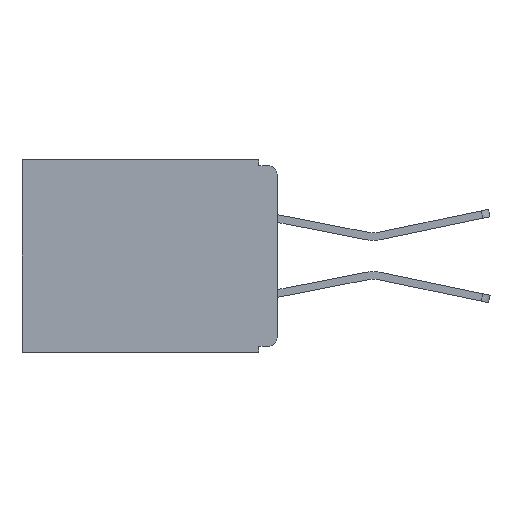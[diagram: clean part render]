
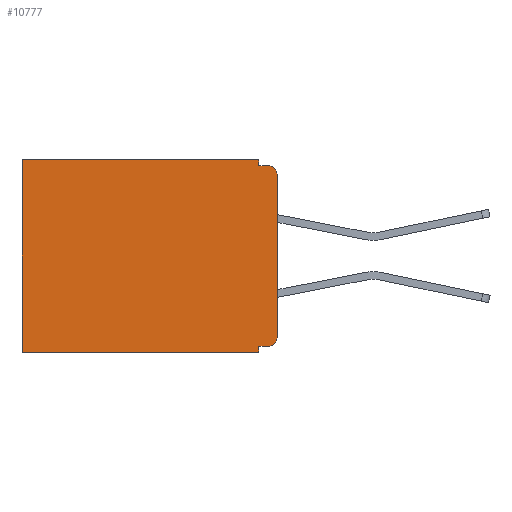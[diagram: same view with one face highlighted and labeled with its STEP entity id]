
A CAD part, left-side view. The second image highlights one B-rep face of the part: STEP entity #10777.
In plain terms, the highlighted planar face has unit normal (-1, 0, 0).
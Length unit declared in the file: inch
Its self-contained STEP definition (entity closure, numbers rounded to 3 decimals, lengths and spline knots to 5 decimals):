
#31 = CARTESIAN_POINT ( 'NONE',  ( 0.3, 0.015, -0.32 ) ) ;
#32 = EDGE_CURVE ( 'NONE', #7214, #6674, #7063, .T. ) ;
#183 = EDGE_CURVE ( 'NONE', #6575, #789, #5731, .T. ) ;
#282 = EDGE_CURVE ( 'NONE', #1045, #8537, #10183, .T. ) ;
#474 = DIRECTION ( 'NONE',  ( 0., 0., -1. ) ) ;
#475 = ORIENTED_EDGE ( 'NONE', *, *, #32, .T. ) ;
#490 = VECTOR ( 'NONE', #5329, 39.37008 ) ;
#765 = LINE ( 'NONE', #10491, #2820 ) ;
#789 = VERTEX_POINT ( 'NONE', #7204 ) ;
#797 = CARTESIAN_POINT ( 'NONE',  ( 0.3, 0., -0.33 ) ) ;
#808 = CARTESIAN_POINT ( 'NONE',  ( 0.3, 0., -0.025 ) ) ;
#1029 = FACE_OUTER_BOUND ( 'NONE', #3842, .T. ) ;
#1045 = VERTEX_POINT ( 'NONE', #3556 ) ;
#1159 = EDGE_CURVE ( 'NONE', #8537, #3041, #9257, .T. ) ;
#1324 = VECTOR ( 'NONE', #3701, 39.37008 ) ;
#1731 = EDGE_CURVE ( 'NONE', #2744, #3041, #5409, .T. ) ;
#2053 = EDGE_CURVE ( 'NONE', #1045, #8242, #10256, .T. ) ;
#2115 = EDGE_CURVE ( 'NONE', #4484, #2744, #765, .T. ) ;
#2306 = ORIENTED_EDGE ( 'NONE', *, *, #183, .T. ) ;
#2744 = VERTEX_POINT ( 'NONE', #6835 ) ;
#2820 = VECTOR ( 'NONE', #8658, 39.37008 ) ;
#3041 = VERTEX_POINT ( 'NONE', #7373 ) ;
#3066 = LINE ( 'NONE', #4452, #490 ) ;
#3301 = ORIENTED_EDGE ( 'NONE', *, *, #1731, .F. ) ;
#3378 = DIRECTION ( 'NONE',  ( 0., 1., 0. ) ) ;
#3556 = CARTESIAN_POINT ( 'NONE',  ( 0.3, 0.031, 0. ) ) ;
#3606 = ORIENTED_EDGE ( 'NONE', *, *, #2053, .F. ) ;
#3701 = DIRECTION ( 'NONE',  ( 0., 0., -1. ) ) ;
#3842 = EDGE_LOOP ( 'NONE', ( #9832, #475, #7612, #3606, #7212, #6824, #3301, #7018, #8519, #2306 ) ) ;
#3924 = PLANE ( 'NONE',  #8973 ) ;
#4018 = LINE ( 'NONE', #4693, #6080 ) ;
#4452 = CARTESIAN_POINT ( 'NONE',  ( 0.3, 0., -0.01 ) ) ;
#4484 = VERTEX_POINT ( 'NONE', #8660 ) ;
#4614 = CARTESIAN_POINT ( 'NONE',  ( 0.3, 0.031, 0. ) ) ;
#4693 = CARTESIAN_POINT ( 'NONE',  ( 0.3, 0., -0.32 ) ) ;
#5157 = CARTESIAN_POINT ( 'NONE',  ( 0.3, 0., 0. ) ) ;
#5329 = DIRECTION ( 'NONE',  ( 0., -1., 0. ) ) ;
#5409 = LINE ( 'NONE', #7278, #7640 ) ;
#5490 = DIRECTION ( 'NONE',  ( 0., 0., -1. ) ) ;
#5549 = DIRECTION ( 'NONE',  ( 0., 1., 0. ) ) ;
#5674 = DIRECTION ( 'NONE',  ( 1., 0., 0. ) ) ;
#5731 = CIRCLE ( 'NONE', #7238, 0.015 ) ;
#5920 = LINE ( 'NONE', #797, #7860 ) ;
#6005 = DIRECTION ( 'NONE',  ( 0., 0., -1. ) ) ;
#6080 = VECTOR ( 'NONE', #5549, 39.37008 ) ;
#6239 = CARTESIAN_POINT ( 'NONE',  ( 0.3, 0.015, -0.305 ) ) ;
#6575 = VERTEX_POINT ( 'NONE', #31 ) ;
#6581 = DIRECTION ( 'NONE',  ( -1., 0., 0. ) ) ;
#6619 = DIRECTION ( 'NONE',  ( 0., 0., -1. ) ) ;
#6654 = CARTESIAN_POINT ( 'NONE',  ( 0.3, 0.437, 0. ) ) ;
#6674 = VERTEX_POINT ( 'NONE', #7114 ) ;
#6824 = ORIENTED_EDGE ( 'NONE', *, *, #1159, .T. ) ;
#6835 = CARTESIAN_POINT ( 'NONE',  ( 0.3, 0.031, -0.33 ) ) ;
#7018 = ORIENTED_EDGE ( 'NONE', *, *, #2115, .F. ) ;
#7063 = CIRCLE ( 'NONE', #10132, 0.015 ) ;
#7114 = CARTESIAN_POINT ( 'NONE',  ( 0.3, 0.015, -0.01 ) ) ;
#7149 = VECTOR ( 'NONE', #5490, 39.37008 ) ;
#7204 = CARTESIAN_POINT ( 'NONE',  ( 0.3, 0., -0.305 ) ) ;
#7212 = ORIENTED_EDGE ( 'NONE', *, *, #282, .T. ) ;
#7214 = VERTEX_POINT ( 'NONE', #808 ) ;
#7235 = CARTESIAN_POINT ( 'NONE',  ( 0.3, 0.031, -0.01 ) ) ;
#7238 = AXIS2_PLACEMENT_3D ( 'NONE', #6239, #6581, #6619 ) ;
#7278 = CARTESIAN_POINT ( 'NONE',  ( 0.3, 0., -0.33 ) ) ;
#7348 = EDGE_CURVE ( 'NONE', #8242, #6674, #3066, .T. ) ;
#7373 = CARTESIAN_POINT ( 'NONE',  ( 0.3, 0.437, -0.33 ) ) ;
#7612 = ORIENTED_EDGE ( 'NONE', *, *, #7348, .F. ) ;
#7640 = VECTOR ( 'NONE', #3378, 39.37008 ) ;
#7789 = CARTESIAN_POINT ( 'NONE',  ( 0.3, 0.437, -0.33 ) ) ;
#7860 = VECTOR ( 'NONE', #6005, 39.37008 ) ;
#8048 = VECTOR ( 'NONE', #8357, 39.37008 ) ;
#8242 = VERTEX_POINT ( 'NONE', #7235 ) ;
#8279 = EDGE_CURVE ( 'NONE', #6575, #4484, #4018, .T. ) ;
#8357 = DIRECTION ( 'NONE',  ( 0., 1., 0. ) ) ;
#8519 = ORIENTED_EDGE ( 'NONE', *, *, #8279, .F. ) ;
#8537 = VERTEX_POINT ( 'NONE', #6654 ) ;
#8658 = DIRECTION ( 'NONE',  ( 0., 0., -1. ) ) ;
#8660 = CARTESIAN_POINT ( 'NONE',  ( 0.3, 0.031, -0.32 ) ) ;
#8973 = AXIS2_PLACEMENT_3D ( 'NONE', #10525, #5674, #474 ) ;
#9257 = LINE ( 'NONE', #7789, #7149 ) ;
#9511 = DIRECTION ( 'NONE',  ( -1., 0., 0. ) ) ;
#9722 = CARTESIAN_POINT ( 'NONE',  ( 0.3, 0.015, -0.025 ) ) ;
#9832 = ORIENTED_EDGE ( 'NONE', *, *, #10114, .F. ) ;
#10114 = EDGE_CURVE ( 'NONE', #7214, #789, #5920, .T. ) ;
#10132 = AXIS2_PLACEMENT_3D ( 'NONE', #9722, #9511, #10157 ) ;
#10157 = DIRECTION ( 'NONE',  ( 0., 0., -1. ) ) ;
#10183 = LINE ( 'NONE', #5157, #8048 ) ;
#10256 = LINE ( 'NONE', #4614, #1324 ) ;
#10491 = CARTESIAN_POINT ( 'NONE',  ( 0.3, 0.031, -0.33 ) ) ;
#10525 = CARTESIAN_POINT ( 'NONE',  ( 0.3, 0., -0.33 ) ) ;
#10777 = ADVANCED_FACE ( 'NONE', ( #1029 ), #3924, .F. ) ;
